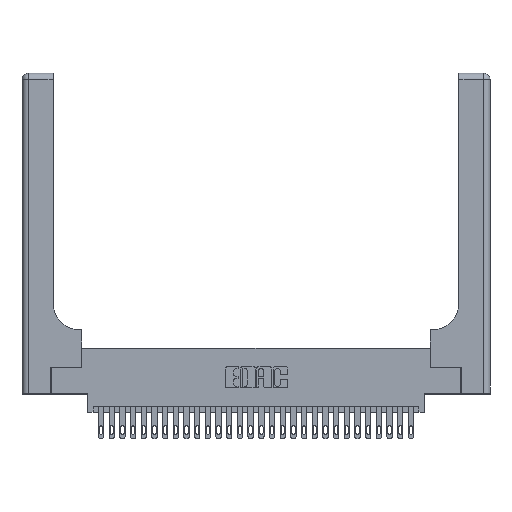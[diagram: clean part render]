
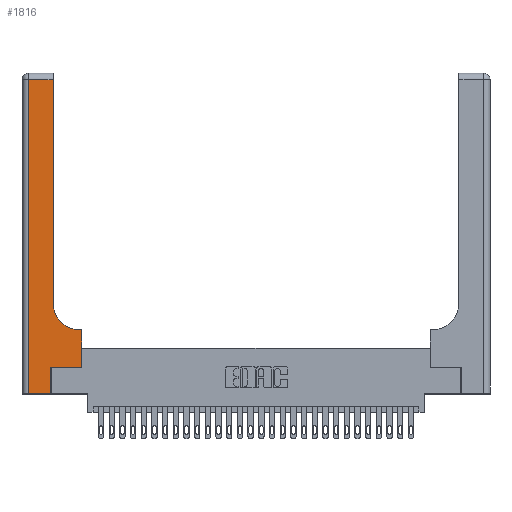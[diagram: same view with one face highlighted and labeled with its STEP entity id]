
A CAD part, top view. The second image highlights one B-rep face of the part: STEP entity #1816.
In plain terms, the highlighted planar face has unit normal (0, 0, 1).
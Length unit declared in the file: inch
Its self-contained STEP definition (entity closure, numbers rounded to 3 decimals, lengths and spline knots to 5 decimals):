
#595 = DIRECTION ( 'NONE',  ( 0., 1., 0. ) ) ;
#1816 = ADVANCED_FACE ( 'NONE', ( #27436 ), #3634, .F. ) ;
#1848 = CARTESIAN_POINT ( 'NONE',  ( 0.2915, 0.85, 0.37 ) ) ;
#2419 = DIRECTION ( 'NONE',  ( 1., 0., 0. ) ) ;
#3510 = CARTESIAN_POINT ( 'NONE',  ( 0.5415, 0.85, 0.37 ) ) ;
#3634 = PLANE ( 'NONE',  #10385 ) ;
#4286 = EDGE_CURVE ( 'NONE', #12330, #28673, #20327, .T. ) ;
#4589 = ORIENTED_EDGE ( 'NONE', *, *, #10218, .T. ) ;
#5734 = DIRECTION ( 'NONE',  ( -1., 0., 0. ) ) ;
#6292 = VECTOR ( 'NONE', #10718, 39.37008 ) ;
#6436 = CARTESIAN_POINT ( 'NONE',  ( 0.269, 0., 0.37 ) ) ;
#6495 = DIRECTION ( 'NONE',  ( -1., 0., 0. ) ) ;
#6693 = LINE ( 'NONE', #17990, #14393 ) ;
#6722 = EDGE_CURVE ( 'NONE', #18919, #20873, #19467, .T. ) ;
#7319 = ORIENTED_EDGE ( 'NONE', *, *, #29862, .T. ) ;
#7548 = DIRECTION ( 'NONE',  ( -1., 0., 0. ) ) ;
#8235 = DIRECTION ( 'NONE',  ( 0., 1., 0. ) ) ;
#8462 = LINE ( 'NONE', #12445, #19459 ) ;
#8954 = VECTOR ( 'NONE', #25596, 39.37008 ) ;
#9370 = EDGE_CURVE ( 'NONE', #20873, #27251, #15220, .T. ) ;
#9541 = LINE ( 'NONE', #21768, #15468 ) ;
#9796 = CARTESIAN_POINT ( 'NONE',  ( 0.5585, 0.25, 0.37 ) ) ;
#10063 = EDGE_LOOP ( 'NONE', ( #7319, #11433, #17850, #10870, #13002, #27419, #25243, #28194, #4589 ) ) ;
#10218 = EDGE_CURVE ( 'NONE', #16289, #15394, #30244, .T. ) ;
#10271 = CARTESIAN_POINT ( 'NONE',  ( 0.5585, 0.6, 0.37 ) ) ;
#10385 = AXIS2_PLACEMENT_3D ( 'NONE', #29507, #22783, #6495 ) ;
#10718 = DIRECTION ( 'NONE',  ( 0., -1., 0. ) ) ;
#10738 = EDGE_CURVE ( 'NONE', #28673, #18919, #15498, .T. ) ;
#10769 = DIRECTION ( 'NONE',  ( 0., 0., -1. ) ) ;
#10870 = ORIENTED_EDGE ( 'NONE', *, *, #6722, .T. ) ;
#11007 = CARTESIAN_POINT ( 'NONE',  ( 0., 0., 0.37 ) ) ;
#11433 = ORIENTED_EDGE ( 'NONE', *, *, #4286, .T. ) ;
#11737 = EDGE_CURVE ( 'NONE', #24204, #12973, #29398, .T. ) ;
#12330 = VERTEX_POINT ( 'NONE', #22230 ) ;
#12445 = CARTESIAN_POINT ( 'NONE',  ( 0.2915, 3., 0.37 ) ) ;
#12973 = VERTEX_POINT ( 'NONE', #10271 ) ;
#13002 = ORIENTED_EDGE ( 'NONE', *, *, #9370, .T. ) ;
#14024 = CARTESIAN_POINT ( 'NONE',  ( 0.5415, 0.6, 0.37 ) ) ;
#14393 = VECTOR ( 'NONE', #27668, 39.37008 ) ;
#15220 = LINE ( 'NONE', #27873, #8954 ) ;
#15394 = VERTEX_POINT ( 'NONE', #1848 ) ;
#15468 = VECTOR ( 'NONE', #7548, 39.37008 ) ;
#15498 = LINE ( 'NONE', #27086, #6292 ) ;
#15918 = CARTESIAN_POINT ( 'NONE',  ( 0.06, 0., 0.37 ) ) ;
#15932 = VECTOR ( 'NONE', #5734, 39.37008 ) ;
#16203 = VECTOR ( 'NONE', #2419, 39.37008 ) ;
#16289 = VERTEX_POINT ( 'NONE', #14024 ) ;
#17850 = ORIENTED_EDGE ( 'NONE', *, *, #10738, .T. ) ;
#17990 = CARTESIAN_POINT ( 'NONE',  ( 0.269, 0.25, 0.37 ) ) ;
#18919 = VERTEX_POINT ( 'NONE', #15918 ) ;
#19173 = AXIS2_PLACEMENT_3D ( 'NONE', #3510, #10769, #25354 ) ;
#19459 = VECTOR ( 'NONE', #8235, 39.37008 ) ;
#19467 = LINE ( 'NONE', #11007, #16203 ) ;
#19473 = CARTESIAN_POINT ( 'NONE',  ( 0.06, 2.94, 0.37 ) ) ;
#19815 = EDGE_CURVE ( 'NONE', #27251, #24204, #6693, .T. ) ;
#20066 = CARTESIAN_POINT ( 'NONE',  ( 0., 2.94, 0.37 ) ) ;
#20327 = LINE ( 'NONE', #20066, #15932 ) ;
#20873 = VERTEX_POINT ( 'NONE', #6436 ) ;
#21388 = CARTESIAN_POINT ( 'NONE',  ( 0.5585, 0.25, 0.37 ) ) ;
#21768 = CARTESIAN_POINT ( 'NONE',  ( 0.2915, 0.6, 0.37 ) ) ;
#22230 = CARTESIAN_POINT ( 'NONE',  ( 0.2915, 2.94, 0.37 ) ) ;
#22783 = DIRECTION ( 'NONE',  ( 0., 0., -1. ) ) ;
#23850 = VECTOR ( 'NONE', #595, 39.37008 ) ;
#24204 = VERTEX_POINT ( 'NONE', #21388 ) ;
#25243 = ORIENTED_EDGE ( 'NONE', *, *, #11737, .T. ) ;
#25354 = DIRECTION ( 'NONE',  ( 1., 0., 0. ) ) ;
#25596 = DIRECTION ( 'NONE',  ( 0., 1., 0. ) ) ;
#26216 = CARTESIAN_POINT ( 'NONE',  ( 0.269, 0.25, 0.37 ) ) ;
#27086 = CARTESIAN_POINT ( 'NONE',  ( 0.06, 3., 0.37 ) ) ;
#27251 = VERTEX_POINT ( 'NONE', #26216 ) ;
#27419 = ORIENTED_EDGE ( 'NONE', *, *, #19815, .T. ) ;
#27436 = FACE_OUTER_BOUND ( 'NONE', #10063, .T. ) ;
#27668 = DIRECTION ( 'NONE',  ( 1., 0., 0. ) ) ;
#27873 = CARTESIAN_POINT ( 'NONE',  ( 0.269, 0., 0.37 ) ) ;
#28194 = ORIENTED_EDGE ( 'NONE', *, *, #29673, .T. ) ;
#28673 = VERTEX_POINT ( 'NONE', #19473 ) ;
#29398 = LINE ( 'NONE', #9796, #23850 ) ;
#29507 = CARTESIAN_POINT ( 'NONE',  ( 0., 3., 0.37 ) ) ;
#29673 = EDGE_CURVE ( 'NONE', #12973, #16289, #9541, .T. ) ;
#29862 = EDGE_CURVE ( 'NONE', #15394, #12330, #8462, .T. ) ;
#30244 = CIRCLE ( 'NONE', #19173, 0.25 ) ;
